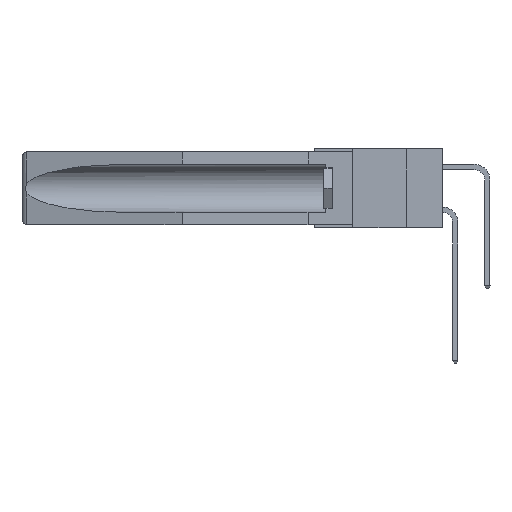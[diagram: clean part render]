
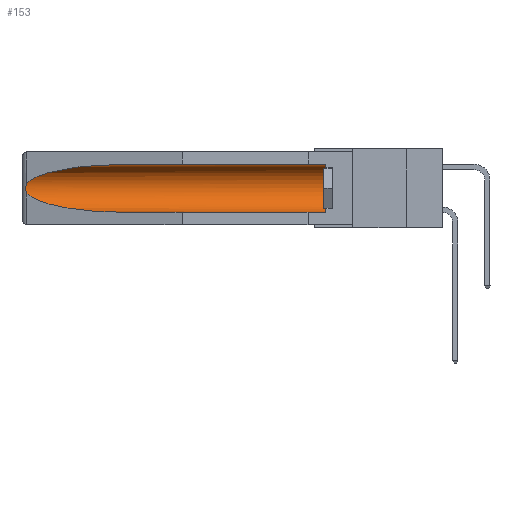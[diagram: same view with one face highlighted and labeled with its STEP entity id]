
A CAD part, left-side view. The second image highlights one B-rep face of the part: STEP entity #153.
In plain terms, the highlighted cylindrical face has radius 2.857 mm (diameter 5.715 mm), a partial arc.
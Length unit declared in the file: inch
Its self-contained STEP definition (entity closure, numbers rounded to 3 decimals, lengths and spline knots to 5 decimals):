
#7 = CARTESIAN_POINT ( 'NONE',  ( 0.155, 1.07973, -0.284 ) ) ;
#153 = ADVANCED_FACE ( 'NONE', ( #19608 ), #6247, .F. ) ;
#236 = ORIENTED_EDGE ( 'NONE', *, *, #4053, .T. ) ;
#295 = CARTESIAN_POINT ( 'NONE',  ( 0.155, -0.30754, -0.059 ) ) ;
#384 = CARTESIAN_POINT ( 'NONE',  ( 0.26537, 1.52718, -0.14972 ) ) ;
#1354 =( BOUNDED_CURVE ( )  B_SPLINE_CURVE ( 3, ( #18026, #5625, #20453, #20292 ),
 .UNSPECIFIED., .F., .F. ) 
 B_SPLINE_CURVE_WITH_KNOTS ( ( 4, 4 ),
 ( 4.71239, 6.08839 ),
 .UNSPECIFIED. ) 
 CURVE ( )  GEOMETRIC_REPRESENTATION_ITEM ( )  RATIONAL_B_SPLINE_CURVE ( ( 1., 0.848, 0.848, 1. ) ) 
 REPRESENTATION_ITEM ( '' )  );
#1884 = EDGE_LOOP ( 'NONE', ( #12219, #2342, #236, #21776, #17437, #8385 ) ) ;
#1948 = CARTESIAN_POINT ( 'NONE',  ( 0.2673, 1.53269, -0.17917 ) ) ;
#2342 = ORIENTED_EDGE ( 'NONE', *, *, #23415, .T. ) ;
#2756 =( BOUNDED_CURVE ( )  B_SPLINE_CURVE ( 3, ( #16639, #22260, #11133, #7 ),
 .UNSPECIFIED., .F., .T. ) 
 B_SPLINE_CURVE_WITH_KNOTS ( ( 4, 4 ),
 ( 0.1948, 1.5708 ),
 .UNSPECIFIED. ) 
 CURVE ( )  GEOMETRIC_REPRESENTATION_ITEM ( )  RATIONAL_B_SPLINE_CURVE ( ( 1., 0.848, 0.848, 1. ) ) 
 REPRESENTATION_ITEM ( '' )  );
#3820 = VERTEX_POINT ( 'NONE', #12136 ) ;
#3884 = B_SPLINE_CURVE_WITH_KNOTS ( 'NONE', 3,
 ( #384, #13193, #20535, #20619, #18798, #22344, #1948, #11449, #13346, #14943 ),
 .UNSPECIFIED., .F., .F.,
 ( 4, 2, 2, 2, 4 ),
 ( 0., 0.00029, 0.00058, 0.00087, 0.00117 ),
 .UNSPECIFIED. ) ;
#4053 = EDGE_CURVE ( 'NONE', #12601, #14172, #2756, .T. ) ;
#4348 = CARTESIAN_POINT ( 'NONE',  ( 0.155, -0.30754, -0.284 ) ) ;
#4542 = LINE ( 'NONE', #4348, #8299 ) ;
#5092 = VERTEX_POINT ( 'NONE', #17862 ) ;
#5625 = CARTESIAN_POINT ( 'NONE',  ( 0.21114, 1.30732, -0.059 ) ) ;
#5819 = EDGE_CURVE ( 'NONE', #5092, #14172, #4542, .T. ) ;
#6247 = CYLINDRICAL_SURFACE ( 'NONE', #17301, 0.1125 ) ;
#8299 = VECTOR ( 'NONE', #18851, 39.37008 ) ;
#8322 = VECTOR ( 'NONE', #11593, 39.37008 ) ;
#8385 = ORIENTED_EDGE ( 'NONE', *, *, #20107, .T. ) ;
#8940 = AXIS2_PLACEMENT_3D ( 'NONE', #10496, #17861, #12301 ) ;
#10496 = CARTESIAN_POINT ( 'NONE',  ( 0.155, 0.126, -0.1715 ) ) ;
#10569 = EDGE_CURVE ( 'NONE', #3820, #18913, #1354, .T. ) ;
#10701 = CARTESIAN_POINT ( 'NONE',  ( 0.155, 1.07973, -0.284 ) ) ;
#11133 = CARTESIAN_POINT ( 'NONE',  ( 0.21114, 1.30732, -0.284 ) ) ;
#11449 = CARTESIAN_POINT ( 'NONE',  ( 0.26655, 1.53094, -0.18657 ) ) ;
#11593 = DIRECTION ( 'NONE',  ( 0., 1., 0. ) ) ;
#12136 = CARTESIAN_POINT ( 'NONE',  ( 0.155, 1.07973, -0.059 ) ) ;
#12219 = ORIENTED_EDGE ( 'NONE', *, *, #10569, .T. ) ;
#12301 = DIRECTION ( 'NONE',  ( 0., 0., 1. ) ) ;
#12509 = CARTESIAN_POINT ( 'NONE',  ( 0.155, 0.126, -0.059 ) ) ;
#12601 = VERTEX_POINT ( 'NONE', #14794 ) ;
#12853 = EDGE_CURVE ( 'NONE', #5092, #19270, #19421, .T. ) ;
#13193 = CARTESIAN_POINT ( 'NONE',  ( 0.26597, 1.52961, -0.15275 ) ) ;
#13346 = CARTESIAN_POINT ( 'NONE',  ( 0.26597, 1.5296, -0.19026 ) ) ;
#14079 = CARTESIAN_POINT ( 'NONE',  ( 0.155, -0.30754, -0.1715 ) ) ;
#14172 = VERTEX_POINT ( 'NONE', #10701 ) ;
#14794 = CARTESIAN_POINT ( 'NONE',  ( 0.26537, 1.52718, -0.19328 ) ) ;
#14943 = CARTESIAN_POINT ( 'NONE',  ( 0.26537, 1.52718, -0.19328 ) ) ;
#16639 = CARTESIAN_POINT ( 'NONE',  ( 0.26537, 1.52718, -0.19328 ) ) ;
#16860 = CARTESIAN_POINT ( 'NONE',  ( 0.26537, 1.52718, -0.14972 ) ) ;
#17301 = AXIS2_PLACEMENT_3D ( 'NONE', #14079, #17704, #17940 ) ;
#17437 = ORIENTED_EDGE ( 'NONE', *, *, #12853, .T. ) ;
#17704 = DIRECTION ( 'NONE',  ( 0., 1., 0. ) ) ;
#17861 = DIRECTION ( 'NONE',  ( 0., -1., 0. ) ) ;
#17862 = CARTESIAN_POINT ( 'NONE',  ( 0.155, 0.126, -0.284 ) ) ;
#17940 = DIRECTION ( 'NONE',  ( 0., 0., 1. ) ) ;
#18026 = CARTESIAN_POINT ( 'NONE',  ( 0.155, 1.07973, -0.059 ) ) ;
#18798 = CARTESIAN_POINT ( 'NONE',  ( 0.2675, 1.53308, -0.16763 ) ) ;
#18851 = DIRECTION ( 'NONE',  ( 0., 1., 0. ) ) ;
#18913 = VERTEX_POINT ( 'NONE', #16860 ) ;
#19270 = VERTEX_POINT ( 'NONE', #12509 ) ;
#19421 = CIRCLE ( 'NONE', #8940, 0.1125 ) ;
#19608 = FACE_OUTER_BOUND ( 'NONE', #1884, .T. ) ;
#20107 = EDGE_CURVE ( 'NONE', #19270, #3820, #23158, .T. ) ;
#20292 = CARTESIAN_POINT ( 'NONE',  ( 0.26537, 1.52718, -0.14972 ) ) ;
#20453 = CARTESIAN_POINT ( 'NONE',  ( 0.25451, 1.48313, -0.09465 ) ) ;
#20535 = CARTESIAN_POINT ( 'NONE',  ( 0.26654, 1.53092, -0.15636 ) ) ;
#20619 = CARTESIAN_POINT ( 'NONE',  ( 0.2673, 1.5327, -0.16383 ) ) ;
#21776 = ORIENTED_EDGE ( 'NONE', *, *, #5819, .F. ) ;
#22260 = CARTESIAN_POINT ( 'NONE',  ( 0.25451, 1.48313, -0.24835 ) ) ;
#22344 = CARTESIAN_POINT ( 'NONE',  ( 0.2675, 1.53308, -0.17534 ) ) ;
#23158 = LINE ( 'NONE', #295, #8322 ) ;
#23415 = EDGE_CURVE ( 'NONE', #18913, #12601, #3884, .T. ) ;
